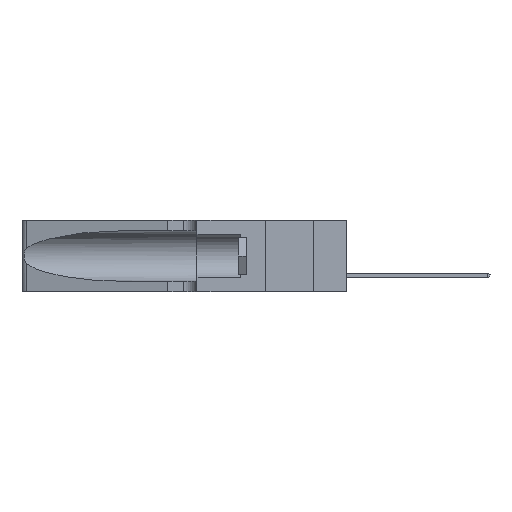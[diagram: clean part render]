
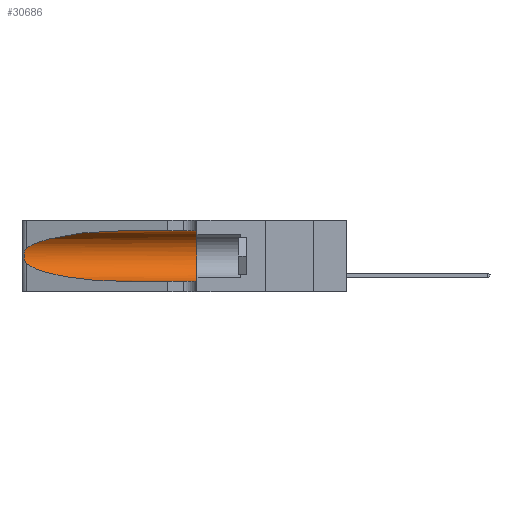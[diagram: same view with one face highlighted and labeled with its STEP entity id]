
A CAD part, left-side view. The second image highlights one B-rep face of the part: STEP entity #30686.
In plain terms, the highlighted cylindrical face has radius 3.308 mm (diameter 6.617 mm), a partial arc.
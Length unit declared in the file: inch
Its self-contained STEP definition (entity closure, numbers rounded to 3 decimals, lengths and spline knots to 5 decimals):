
#24 = CARTESIAN_POINT ( 'NONE',  ( 0.26075, 1.23896, 0.178 ) ) ;
#311 = CARTESIAN_POINT ( 'NONE',  ( 0.25789, 1.23486, 0.15765 ) ) ;
#423 = CARTESIAN_POINT ( 'NONE',  ( 0.25487, 1.22718, 0.22369 ) ) ;
#1069 = DIRECTION ( 'NONE',  ( 0., -1., 0. ) ) ;
#1409 = DIRECTION ( 'NONE',  ( 0., -1., 0. ) ) ;
#1660 = VERTEX_POINT ( 'NONE', #17716 ) ;
#2524 = LINE ( 'NONE', #9464, #2938 ) ;
#2829 = CARTESIAN_POINT ( 'NONE',  ( 0.1305, 0.72297, 0.31525 ) ) ;
#2938 = VECTOR ( 'NONE', #1069, 39.37008 ) ;
#3226 = CARTESIAN_POINT ( 'NONE',  ( 0.26075, 1.23896, 0.19203 ) ) ;
#3298 = VERTEX_POINT ( 'NONE', #25301 ) ;
#3305 = CARTESIAN_POINT ( 'NONE',  ( 0.1305, 1.61858, 0.185 ) ) ;
#3998 = VECTOR ( 'NONE', #1409, 39.37008 ) ;
#4946 = ORIENTED_EDGE ( 'NONE', *, *, #26813, .F. ) ;
#5049 =( BOUNDED_CURVE ( )  B_SPLINE_CURVE ( 3, ( #27884, #11420, #14410, #14538 ),
 .UNSPECIFIED., .F., .T. ) 
 B_SPLINE_CURVE_WITH_KNOTS ( ( 4, 4 ),
 ( 3.44316, 4.71239 ),
 .UNSPECIFIED. ) 
 CURVE ( )  GEOMETRIC_REPRESENTATION_ITEM ( )  RATIONAL_B_SPLINE_CURVE ( ( 1., 0.87, 0.87, 1. ) ) 
 REPRESENTATION_ITEM ( '' )  );
#5548 = EDGE_LOOP ( 'NONE', ( #29083, #20967, #11884, #20492, #4946, #35117 ) ) ;
#5614 = CARTESIAN_POINT ( 'NONE',  ( 0.25555, 1.22993, 0.14849 ) ) ;
#5681 = CIRCLE ( 'NONE', #27401, 0.13025 ) ;
#5719 = CARTESIAN_POINT ( 'NONE',  ( 0.25787, 1.23484, 0.2124 ) ) ;
#7281 = CYLINDRICAL_SURFACE ( 'NONE', #24504, 0.13025 ) ;
#7908 = CARTESIAN_POINT ( 'NONE',  ( 0.18966, 0.96281, 0.31525 ) ) ;
#8599 = CARTESIAN_POINT ( 'NONE',  ( 0.26018, 1.23835, 0.19895 ) ) ;
#8667 = VERTEX_POINT ( 'NONE', #28426 ) ;
#9464 = CARTESIAN_POINT ( 'NONE',  ( 0.1305, 1.61858, 0.05475 ) ) ;
#10794 = DIRECTION ( 'NONE',  ( 0., 0., -1. ) ) ;
#11260 = LINE ( 'NONE', #23348, #3998 ) ;
#11420 = CARTESIAN_POINT ( 'NONE',  ( 0.2373, 1.15595, 0.08982 ) ) ;
#11884 = ORIENTED_EDGE ( 'NONE', *, *, #34275, .T. ) ;
#13315 = CARTESIAN_POINT ( 'NONE',  ( 0.1305, 0.72297, 0.31525 ) ) ;
#14060 = FACE_OUTER_BOUND ( 'NONE', #5548, .T. ) ;
#14110 = CARTESIAN_POINT ( 'NONE',  ( 0.25854, 1.2359, 0.20912 ) ) ;
#14410 = CARTESIAN_POINT ( 'NONE',  ( 0.18966, 0.96281, 0.05475 ) ) ;
#14538 = CARTESIAN_POINT ( 'NONE',  ( 0.1305, 0.72297, 0.05475 ) ) ;
#15392 = B_SPLINE_CURVE_WITH_KNOTS ( 'NONE', 3,
 ( #423, #27607, #19241, #5719, #14110, #8599, #3226, #24, #32925, #24863, #311, #33027, #5614, #22241 ),
 .UNSPECIFIED., .F., .F.,
 ( 4, 2, 2, 2, 2, 2, 4 ),
 ( 0., 0.00027, 0.00053, 0.00107, 0.0016, 0.00187, 0.00214 ),
 .UNSPECIFIED. ) ;
#15422 = VERTEX_POINT ( 'NONE', #24779 ) ;
#17259 = EDGE_CURVE ( 'NONE', #15422, #3298, #2524, .T. ) ;
#17672 = VERTEX_POINT ( 'NONE', #31686 ) ;
#17716 = CARTESIAN_POINT ( 'NONE',  ( 0.25487, 1.22718, 0.14631 ) ) ;
#19241 = CARTESIAN_POINT ( 'NONE',  ( 0.25639, 1.23184, 0.21858 ) ) ;
#20492 = ORIENTED_EDGE ( 'NONE', *, *, #17259, .T. ) ;
#20815 = CARTESIAN_POINT ( 'NONE',  ( 0.1305, 0.35, 0.185 ) ) ;
#20967 = ORIENTED_EDGE ( 'NONE', *, *, #29962, .T. ) ;
#22241 = CARTESIAN_POINT ( 'NONE',  ( 0.25487, 1.22718, 0.14631 ) ) ;
#23348 = CARTESIAN_POINT ( 'NONE',  ( 0.1305, 1.61858, 0.31525 ) ) ;
#24091 = VERTEX_POINT ( 'NONE', #2829 ) ;
#24503 = DIRECTION ( 'NONE',  ( 0., -1., 0. ) ) ;
#24504 = AXIS2_PLACEMENT_3D ( 'NONE', #3305, #24503, #10794 ) ;
#24779 = CARTESIAN_POINT ( 'NONE',  ( 0.1305, 0.72297, 0.05475 ) ) ;
#24863 = CARTESIAN_POINT ( 'NONE',  ( 0.25856, 1.23593, 0.16098 ) ) ;
#24923 = CARTESIAN_POINT ( 'NONE',  ( 0.2373, 1.15595, 0.28018 ) ) ;
#25301 = CARTESIAN_POINT ( 'NONE',  ( 0.1305, 0.35, 0.05475 ) ) ;
#26548 = DIRECTION ( 'NONE',  ( 0., 1., 0. ) ) ;
#26813 = EDGE_CURVE ( 'NONE', #8667, #3298, #5681, .T. ) ;
#26925 =( BOUNDED_CURVE ( )  B_SPLINE_CURVE ( 3, ( #13315, #7908, #24923, #30215 ),
 .UNSPECIFIED., .F., .F. ) 
 B_SPLINE_CURVE_WITH_KNOTS ( ( 4, 4 ),
 ( 1.5708, 2.84003 ),
 .UNSPECIFIED. ) 
 CURVE ( )  GEOMETRIC_REPRESENTATION_ITEM ( )  RATIONAL_B_SPLINE_CURVE ( ( 1., 0.87, 0.87, 1. ) ) 
 REPRESENTATION_ITEM ( '' )  );
#27046 = EDGE_CURVE ( 'NONE', #24091, #17672, #26925, .T. ) ;
#27401 = AXIS2_PLACEMENT_3D ( 'NONE', #20815, #26548, #34918 ) ;
#27607 = CARTESIAN_POINT ( 'NONE',  ( 0.25555, 1.22994, 0.2215 ) ) ;
#27884 = CARTESIAN_POINT ( 'NONE',  ( 0.25487, 1.22718, 0.14631 ) ) ;
#28426 = CARTESIAN_POINT ( 'NONE',  ( 0.1305, 0.35, 0.31525 ) ) ;
#29083 = ORIENTED_EDGE ( 'NONE', *, *, #27046, .T. ) ;
#29962 = EDGE_CURVE ( 'NONE', #17672, #1660, #15392, .T. ) ;
#30215 = CARTESIAN_POINT ( 'NONE',  ( 0.25487, 1.22718, 0.22369 ) ) ;
#30686 = ADVANCED_FACE ( 'NONE', ( #14060 ), #7281, .F. ) ;
#31686 = CARTESIAN_POINT ( 'NONE',  ( 0.25487, 1.22718, 0.22369 ) ) ;
#32925 = CARTESIAN_POINT ( 'NONE',  ( 0.26017, 1.23833, 0.17102 ) ) ;
#33027 = CARTESIAN_POINT ( 'NONE',  ( 0.25639, 1.23186, 0.15144 ) ) ;
#33776 = EDGE_CURVE ( 'NONE', #24091, #8667, #11260, .T. ) ;
#34275 = EDGE_CURVE ( 'NONE', #1660, #15422, #5049, .T. ) ;
#34918 = DIRECTION ( 'NONE',  ( 0., 0., 1. ) ) ;
#35117 = ORIENTED_EDGE ( 'NONE', *, *, #33776, .F. ) ;
